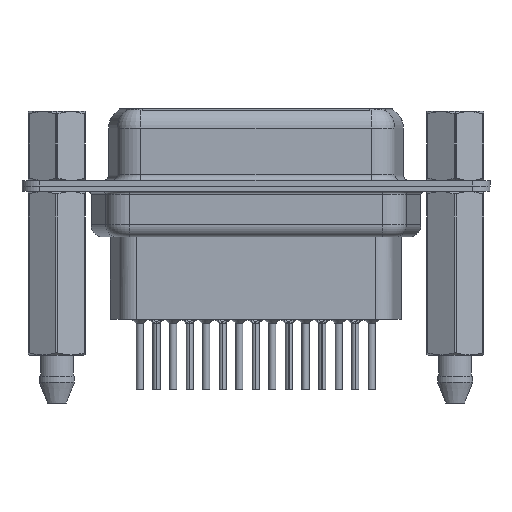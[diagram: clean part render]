
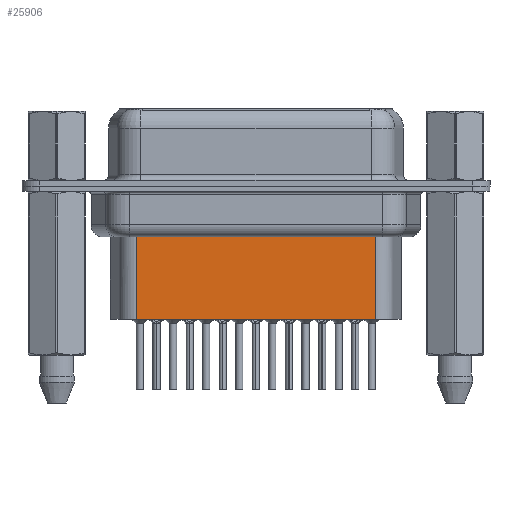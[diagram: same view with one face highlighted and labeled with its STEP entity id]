
A CAD part, front view. The second image highlights one B-rep face of the part: STEP entity #25906.
In plain terms, the highlighted planar face has unit normal (0, -1, 0).
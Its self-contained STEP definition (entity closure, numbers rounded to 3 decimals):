
#65 = DIRECTION ( 'NONE',  ( -1., 0., 0. ) ) ;
#318 = EDGE_LOOP ( 'NONE', ( #3916, #16804, #19856, #2046 ) ) ;
#525 = DIRECTION ( 'NONE',  ( 0., 0., -1. ) ) ;
#767 = CARTESIAN_POINT ( 'NONE',  ( 6.434, -3.5, -4.097 ) ) ;
#1319 = DIRECTION ( 'NONE',  ( 1., 0., 0. ) ) ;
#1462 = LINE ( 'NONE', #767, #25559 ) ;
#2046 = ORIENTED_EDGE ( 'NONE', *, *, #11987, .F. ) ;
#2470 = CARTESIAN_POINT ( 'NONE',  ( 26.619, -3.5, -11.15 ) ) ;
#3619 = VECTOR ( 'NONE', #65, 1000. ) ;
#3916 = ORIENTED_EDGE ( 'NONE', *, *, #23936, .F. ) ;
#4405 = CARTESIAN_POINT ( 'NONE',  ( 26.619, -3.5, -4.097 ) ) ;
#5711 = LINE ( 'NONE', #12713, #18907 ) ;
#6577 = AXIS2_PLACEMENT_3D ( 'NONE', #17706, #29327, #1319 ) ;
#6737 = LINE ( 'NONE', #16624, #18163 ) ;
#7107 = VERTEX_POINT ( 'NONE', #4405 ) ;
#7358 = EDGE_CURVE ( 'NONE', #7107, #23799, #1462, .T. ) ;
#8049 = VERTEX_POINT ( 'NONE', #11892 ) ;
#11622 = CARTESIAN_POINT ( 'NONE',  ( 6.681, -3.5, -11.15 ) ) ;
#11892 = CARTESIAN_POINT ( 'NONE',  ( 6.681, -3.5, -11.15 ) ) ;
#11987 = EDGE_CURVE ( 'NONE', #25357, #8049, #23125, .T. ) ;
#12713 = CARTESIAN_POINT ( 'NONE',  ( 6.681, -3.5, -3.1 ) ) ;
#16392 = EDGE_CURVE ( 'NONE', #23799, #8049, #5711, .T. ) ;
#16624 = CARTESIAN_POINT ( 'NONE',  ( 26.619, -3.5, -3.1 ) ) ;
#16804 = ORIENTED_EDGE ( 'NONE', *, *, #7358, .T. ) ;
#17706 = CARTESIAN_POINT ( 'NONE',  ( 6.681, -3.5, -3.1 ) ) ;
#17844 = CARTESIAN_POINT ( 'NONE',  ( 6.681, -3.5, -4.097 ) ) ;
#18163 = VECTOR ( 'NONE', #525, 1000. ) ;
#18907 = VECTOR ( 'NONE', #19669, 1000. ) ;
#19669 = DIRECTION ( 'NONE',  ( 0., 0., -1. ) ) ;
#19856 = ORIENTED_EDGE ( 'NONE', *, *, #16392, .T. ) ;
#21955 = PLANE ( 'NONE',  #6577 ) ;
#23125 = LINE ( 'NONE', #11622, #3619 ) ;
#23799 = VERTEX_POINT ( 'NONE', #17844 ) ;
#23936 = EDGE_CURVE ( 'NONE', #7107, #25357, #6737, .T. ) ;
#24679 = FACE_OUTER_BOUND ( 'NONE', #318, .T. ) ;
#25357 = VERTEX_POINT ( 'NONE', #2470 ) ;
#25559 = VECTOR ( 'NONE', #27050, 1000. ) ;
#25906 = ADVANCED_FACE ( 'NONE', ( #24679 ), #21955, .T. ) ;
#27050 = DIRECTION ( 'NONE',  ( -1., 0., 0. ) ) ;
#29327 = DIRECTION ( 'NONE',  ( 0., -1., 0. ) ) ;
